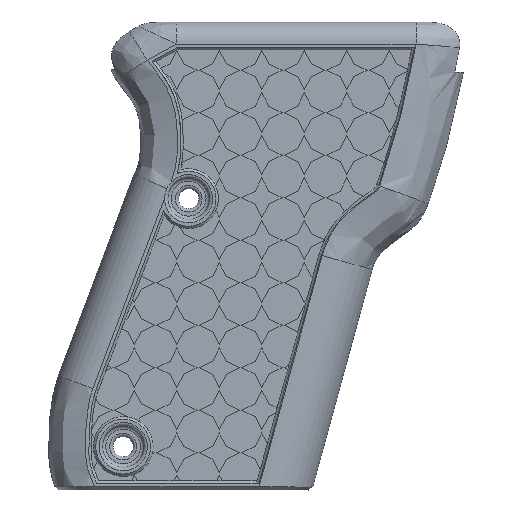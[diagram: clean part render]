
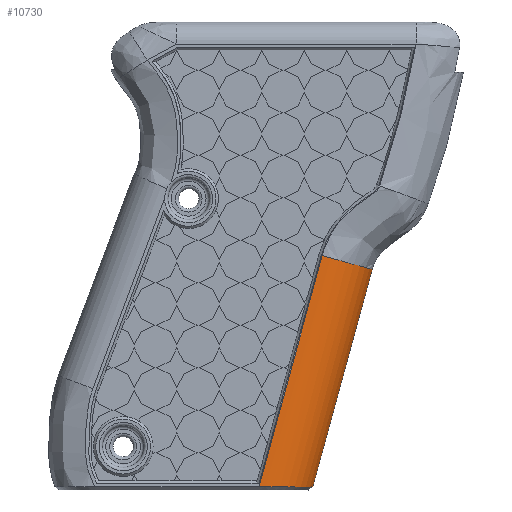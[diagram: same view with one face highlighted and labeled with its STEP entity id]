
A CAD part, front view. The second image highlights one B-rep face of the part: STEP entity #10730.
In plain terms, the highlighted cylindrical face has radius 8 mm (diameter 16 mm), a partial arc.
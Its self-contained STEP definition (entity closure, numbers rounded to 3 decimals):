
#40=CYLINDRICAL_SURFACE('',#11333,8.);
#144=CIRCLE('',#11334,8.);
#1190=FACE_OUTER_BOUND('',#1793,.T.);
#1793=EDGE_LOOP('',(#9932,#9933,#9934,#9935));
#3047=LINE('',#18276,#4362);
#3094=LINE('',#19841,#4409);
#4362=VECTOR('',#13564,8.);
#4409=VECTOR('',#13747,10.);
#4571=B_SPLINE_CURVE_WITH_KNOTS('',3,(#19514,#19515,#19516,#19517,#19518),
 .UNSPECIFIED.,.F.,.F.,(4,1,4),(-6.035,-5.475,-4.729),
 .UNSPECIFIED.);
#5451=VERTEX_POINT('',#18273);
#5452=VERTEX_POINT('',#18275);
#5526=VERTEX_POINT('',#19512);
#5530=VERTEX_POINT('',#19840);
#6900=EDGE_CURVE('',#5452,#5451,#3047,.T.);
#7008=EDGE_CURVE('',#5526,#5451,#4571,.T.);
#7016=EDGE_CURVE('',#5526,#5530,#3094,.T.);
#7017=EDGE_CURVE('',#5530,#5452,#144,.T.);
#9932=ORIENTED_EDGE('',*,*,#7008,.F.);
#9933=ORIENTED_EDGE('',*,*,#7016,.T.);
#9934=ORIENTED_EDGE('',*,*,#7017,.T.);
#9935=ORIENTED_EDGE('',*,*,#6900,.T.);
#10730=ADVANCED_FACE('',(#1190),#40,.T.);
#11333=AXIS2_PLACEMENT_3D('',#19839,#13745,#13746);
#11334=AXIS2_PLACEMENT_3D('',#19842,#13748,#13749);
#13564=DIRECTION('',(-0.264,0.,-0.965));
#13745=DIRECTION('center_axis',(-0.264,0.,-0.965));
#13746=DIRECTION('ref_axis',(0.934,-0.25,-0.255));
#13747=DIRECTION('',(0.264,0.,0.965));
#13748=DIRECTION('center_axis',(-0.264,0.,
-0.965));
#13749=DIRECTION('ref_axis',(0.934,-0.25,-0.255));
#18273=CARTESIAN_POINT('',(13.109,-6.,-36.82));
#18275=CARTESIAN_POINT('',(22.536,-6.,-2.313));
#18276=CARTESIAN_POINT('',(13.53,-6.,-35.279));
#19512=CARTESIAN_POINT('',(21.134,0.,-36.837));
#19514=CARTESIAN_POINT('Ctrl Pts',(21.134,0.,
-36.837));
#19515=CARTESIAN_POINT('Ctrl Pts',(20.741,-1.469,-36.835));
#19516=CARTESIAN_POINT('Ctrl Pts',(18.789,-4.634,-36.827));
#19517=CARTESIAN_POINT('Ctrl Pts',(15.172,-6.,-36.82));
#19518=CARTESIAN_POINT('Ctrl Pts',(13.109,-6.,-36.82));
#19839=CARTESIAN_POINT('Origin',(13.53,2.,-35.279));
#19840=CARTESIAN_POINT('',(30.008,0.,-4.354));
#19841=CARTESIAN_POINT('',(21.002,0.,-37.32));
#19842=CARTESIAN_POINT('Origin',(22.536,2.,-2.313));
